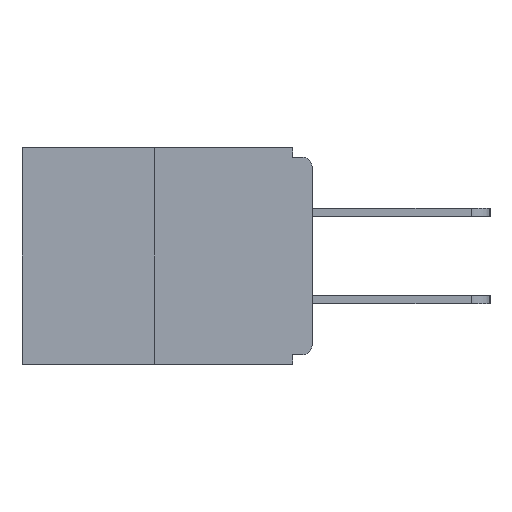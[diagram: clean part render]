
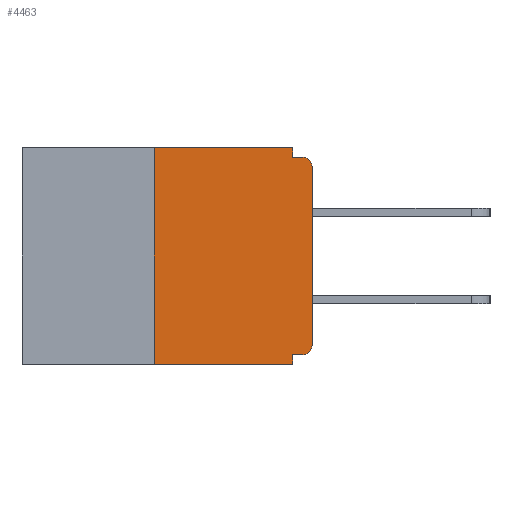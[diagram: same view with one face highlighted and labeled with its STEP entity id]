
A CAD part, left-side view. The second image highlights one B-rep face of the part: STEP entity #4463.
In plain terms, the highlighted planar face has unit normal (-1, 0, 0).
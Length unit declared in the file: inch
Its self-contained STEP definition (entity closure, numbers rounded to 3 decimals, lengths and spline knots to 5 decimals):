
#218 = DIRECTION ( 'NONE',  ( 0., 1., 0. ) ) ;
#857 = EDGE_CURVE ( 'NONE', #13176, #8633, #8752, .T. ) ;
#1006 = CARTESIAN_POINT ( 'NONE',  ( 0., 0.031, -0.343 ) ) ;
#1049 = DIRECTION ( 'NONE',  ( 0., 0., 1. ) ) ;
#1235 = CARTESIAN_POINT ( 'NONE',  ( 0., 0., -0.313 ) ) ;
#1481 = VERTEX_POINT ( 'NONE', #13500 ) ;
#1761 = CARTESIAN_POINT ( 'NONE',  ( 0., 0., -0.03 ) ) ;
#1835 = EDGE_CURVE ( 'NONE', #14061, #12851, #12627, .T. ) ;
#2327 = LINE ( 'NONE', #8489, #12693 ) ;
#2390 = VECTOR ( 'NONE', #15132, 39.37008 ) ;
#3162 = EDGE_LOOP ( 'NONE', ( #17151, #6548, #17365, #4007, #6271, #5816, #3248, #11826, #13720, #15311 ) ) ;
#3248 = ORIENTED_EDGE ( 'NONE', *, *, #6310, .T. ) ;
#3418 = VERTEX_POINT ( 'NONE', #15089 ) ;
#3548 = LINE ( 'NONE', #10401, #15013 ) ;
#4007 = ORIENTED_EDGE ( 'NONE', *, *, #4017, .F. ) ;
#4017 = EDGE_CURVE ( 'NONE', #1481, #8633, #13167, .T. ) ;
#4463 = ADVANCED_FACE ( 'NONE', ( #6725 ), #14177, .F. ) ;
#5091 = CARTESIAN_POINT ( 'NONE',  ( 0., 0.031, -0.343 ) ) ;
#5122 = VERTEX_POINT ( 'NONE', #12993 ) ;
#5816 = ORIENTED_EDGE ( 'NONE', *, *, #1835, .T. ) ;
#5912 = CARTESIAN_POINT ( 'NONE',  ( 0., 0.46, 0. ) ) ;
#6203 = EDGE_CURVE ( 'NONE', #9082, #3418, #11800, .T. ) ;
#6271 = ORIENTED_EDGE ( 'NONE', *, *, #7743, .F. ) ;
#6310 = EDGE_CURVE ( 'NONE', #12851, #17582, #10929, .T. ) ;
#6398 = CARTESIAN_POINT ( 'NONE',  ( 0., 0., -0.015 ) ) ;
#6426 = EDGE_CURVE ( 'NONE', #3418, #8069, #7431, .T. ) ;
#6548 = ORIENTED_EDGE ( 'NONE', *, *, #12808, .F. ) ;
#6725 = FACE_OUTER_BOUND ( 'NONE', #3162, .T. ) ;
#7375 = CARTESIAN_POINT ( 'NONE',  ( 0., 0.015, -0.313 ) ) ;
#7431 = LINE ( 'NONE', #6398, #9377 ) ;
#7743 = EDGE_CURVE ( 'NONE', #14061, #1481, #2327, .T. ) ;
#7966 = CARTESIAN_POINT ( 'NONE',  ( 0., 0.031, 0. ) ) ;
#8069 = VERTEX_POINT ( 'NONE', #9285 ) ;
#8093 = DIRECTION ( 'NONE',  ( 0., 0., -1. ) ) ;
#8114 = DIRECTION ( 'NONE',  ( 0., 0., 1. ) ) ;
#8262 = AXIS2_PLACEMENT_3D ( 'NONE', #7375, #17028, #12773 ) ;
#8489 = CARTESIAN_POINT ( 'NONE',  ( 0., 0., -0.328 ) ) ;
#8633 = VERTEX_POINT ( 'NONE', #1006 ) ;
#8730 = DIRECTION ( 'NONE',  ( 0., 0., -1. ) ) ;
#8752 = LINE ( 'NONE', #14702, #12245 ) ;
#8954 = VECTOR ( 'NONE', #13255, 39.37008 ) ;
#9082 = VERTEX_POINT ( 'NONE', #7966 ) ;
#9285 = CARTESIAN_POINT ( 'NONE',  ( 0., 0.015, -0.015 ) ) ;
#9377 = VECTOR ( 'NONE', #16058, 39.37008 ) ;
#10401 = CARTESIAN_POINT ( 'NONE',  ( 0., 0.46, 0. ) ) ;
#10929 = LINE ( 'NONE', #15137, #11347 ) ;
#11347 = VECTOR ( 'NONE', #8114, 39.37008 ) ;
#11571 = LINE ( 'NONE', #13413, #15690 ) ;
#11800 = LINE ( 'NONE', #12136, #8954 ) ;
#11826 = ORIENTED_EDGE ( 'NONE', *, *, #14445, .T. ) ;
#12136 = CARTESIAN_POINT ( 'NONE',  ( 0., 0.031, 0. ) ) ;
#12245 = VECTOR ( 'NONE', #13693, 39.37008 ) ;
#12275 = CARTESIAN_POINT ( 'NONE',  ( 0., 0.25, -0.343 ) ) ;
#12289 = DIRECTION ( 'NONE',  ( -1., 0., 0. ) ) ;
#12627 = CIRCLE ( 'NONE', #8262, 0.015 ) ;
#12693 = VECTOR ( 'NONE', #218, 39.37008 ) ;
#12773 = DIRECTION ( 'NONE',  ( 0., 0., -1. ) ) ;
#12808 = EDGE_CURVE ( 'NONE', #13176, #5122, #11571, .T. ) ;
#12851 = VERTEX_POINT ( 'NONE', #1235 ) ;
#12993 = CARTESIAN_POINT ( 'NONE',  ( 0., 0.25, 0. ) ) ;
#13167 = LINE ( 'NONE', #5091, #2390 ) ;
#13176 = VERTEX_POINT ( 'NONE', #12275 ) ;
#13255 = DIRECTION ( 'NONE',  ( 0., 0., -1. ) ) ;
#13413 = CARTESIAN_POINT ( 'NONE',  ( 0., 0.25, 0. ) ) ;
#13500 = CARTESIAN_POINT ( 'NONE',  ( 0., 0.031, -0.328 ) ) ;
#13693 = DIRECTION ( 'NONE',  ( 0., -1., 0. ) ) ;
#13713 = CIRCLE ( 'NONE', #17786, 0.015 ) ;
#13720 = ORIENTED_EDGE ( 'NONE', *, *, #6426, .F. ) ;
#14061 = VERTEX_POINT ( 'NONE', #17353 ) ;
#14177 = PLANE ( 'NONE',  #15594 ) ;
#14385 = EDGE_CURVE ( 'NONE', #5122, #9082, #3548, .T. ) ;
#14445 = EDGE_CURVE ( 'NONE', #17582, #8069, #13713, .T. ) ;
#14702 = CARTESIAN_POINT ( 'NONE',  ( 0., 0.46, -0.343 ) ) ;
#14876 = CARTESIAN_POINT ( 'NONE',  ( 0., 0.015, -0.03 ) ) ;
#15013 = VECTOR ( 'NONE', #15956, 39.37008 ) ;
#15089 = CARTESIAN_POINT ( 'NONE',  ( 0., 0.031, -0.015 ) ) ;
#15132 = DIRECTION ( 'NONE',  ( 0., 0., -1. ) ) ;
#15137 = CARTESIAN_POINT ( 'NONE',  ( 0., 0., 0. ) ) ;
#15311 = ORIENTED_EDGE ( 'NONE', *, *, #6203, .F. ) ;
#15580 = DIRECTION ( 'NONE',  ( 1., 0., 0. ) ) ;
#15594 = AXIS2_PLACEMENT_3D ( 'NONE', #5912, #15580, #8730 ) ;
#15690 = VECTOR ( 'NONE', #1049, 39.37008 ) ;
#15956 = DIRECTION ( 'NONE',  ( 0., -1., 0. ) ) ;
#16058 = DIRECTION ( 'NONE',  ( 0., -1., 0. ) ) ;
#17028 = DIRECTION ( 'NONE',  ( -1., 0., 0. ) ) ;
#17151 = ORIENTED_EDGE ( 'NONE', *, *, #14385, .F. ) ;
#17353 = CARTESIAN_POINT ( 'NONE',  ( 0., 0.015, -0.328 ) ) ;
#17365 = ORIENTED_EDGE ( 'NONE', *, *, #857, .T. ) ;
#17582 = VERTEX_POINT ( 'NONE', #1761 ) ;
#17786 = AXIS2_PLACEMENT_3D ( 'NONE', #14876, #12289, #8093 ) ;
